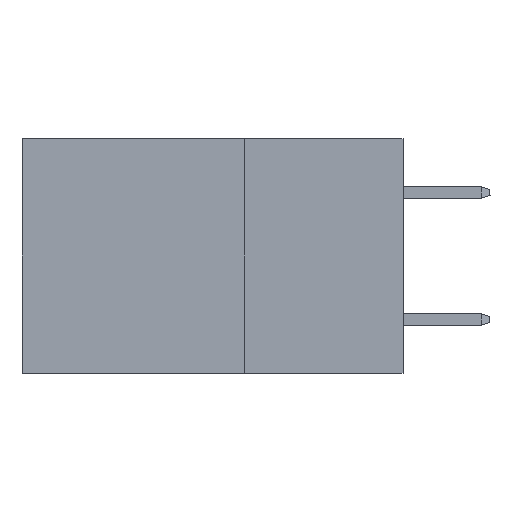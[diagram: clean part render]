
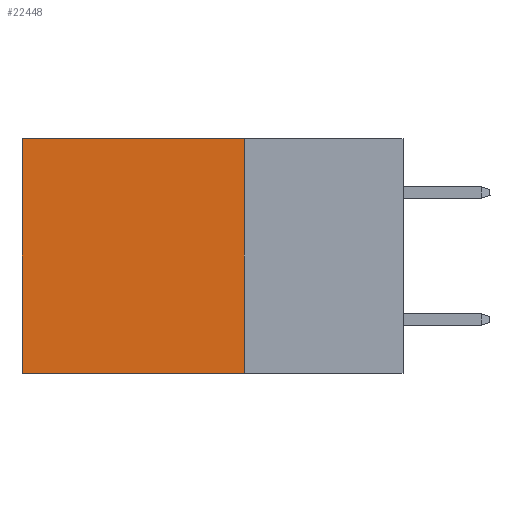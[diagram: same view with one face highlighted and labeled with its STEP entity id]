
A CAD part, left-side view. The second image highlights one B-rep face of the part: STEP entity #22448.
In plain terms, the highlighted planar face has unit normal (-1, 0, 0).
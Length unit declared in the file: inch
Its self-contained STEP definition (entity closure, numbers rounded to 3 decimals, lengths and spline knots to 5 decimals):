
#1595 = ORIENTED_EDGE ( 'NONE', *, *, #27881, .T. ) ;
#2287 = CARTESIAN_POINT ( 'NONE',  ( 0.2875, 0.25, 0. ) ) ;
#4432 = ORIENTED_EDGE ( 'NONE', *, *, #30291, .F. ) ;
#5295 = VECTOR ( 'NONE', #37711, 39.37008 ) ;
#5941 = VECTOR ( 'NONE', #10640, 39.37008 ) ;
#6083 = PLANE ( 'NONE',  #23229 ) ;
#6540 = CARTESIAN_POINT ( 'NONE',  ( 0.2875, 0.25, 0. ) ) ;
#7558 = LINE ( 'NONE', #22466, #5941 ) ;
#10640 = DIRECTION ( 'NONE',  ( 0., 1., 0. ) ) ;
#11552 = EDGE_CURVE ( 'NONE', #40549, #23185, #7558, .T. ) ;
#12274 = LINE ( 'NONE', #26729, #29197 ) ;
#12693 = VERTEX_POINT ( 'NONE', #29727 ) ;
#13876 = DIRECTION ( 'NONE',  ( 0., 0., -1. ) ) ;
#15910 = LINE ( 'NONE', #30406, #5295 ) ;
#18132 = CARTESIAN_POINT ( 'NONE',  ( 0.2875, 0.25, -0.37 ) ) ;
#18341 = DIRECTION ( 'NONE',  ( 0., 0., -1. ) ) ;
#18804 = LINE ( 'NONE', #36342, #38723 ) ;
#20341 = CARTESIAN_POINT ( 'NONE',  ( 0.2875, 0.6, 0. ) ) ;
#20693 = EDGE_CURVE ( 'NONE', #29151, #12693, #12274, .T. ) ;
#22448 = ADVANCED_FACE ( 'NONE', ( #23846 ), #6083, .F. ) ;
#22466 = CARTESIAN_POINT ( 'NONE',  ( 0.2875, 0.25, 0. ) ) ;
#23185 = VERTEX_POINT ( 'NONE', #20341 ) ;
#23229 = AXIS2_PLACEMENT_3D ( 'NONE', #6540, #34737, #13876 ) ;
#23846 = FACE_OUTER_BOUND ( 'NONE', #38340, .T. ) ;
#26729 = CARTESIAN_POINT ( 'NONE',  ( 0.2875, 0.25, -0.37 ) ) ;
#27881 = EDGE_CURVE ( 'NONE', #23185, #12693, #15910, .T. ) ;
#29151 = VERTEX_POINT ( 'NONE', #18132 ) ;
#29197 = VECTOR ( 'NONE', #41614, 39.37008 ) ;
#29727 = CARTESIAN_POINT ( 'NONE',  ( 0.2875, 0.6, -0.37 ) ) ;
#30291 = EDGE_CURVE ( 'NONE', #40549, #29151, #18804, .T. ) ;
#30406 = CARTESIAN_POINT ( 'NONE',  ( 0.2875, 0.6, 0. ) ) ;
#34621 = ORIENTED_EDGE ( 'NONE', *, *, #20693, .F. ) ;
#34737 = DIRECTION ( 'NONE',  ( 1., 0., 0. ) ) ;
#36342 = CARTESIAN_POINT ( 'NONE',  ( 0.2875, 0.25, 0. ) ) ;
#37711 = DIRECTION ( 'NONE',  ( 0., 0., -1. ) ) ;
#38340 = EDGE_LOOP ( 'NONE', ( #1595, #34621, #4432, #41462 ) ) ;
#38723 = VECTOR ( 'NONE', #18341, 39.37008 ) ;
#40549 = VERTEX_POINT ( 'NONE', #2287 ) ;
#41462 = ORIENTED_EDGE ( 'NONE', *, *, #11552, .T. ) ;
#41614 = DIRECTION ( 'NONE',  ( 0., 1., 0. ) ) ;
